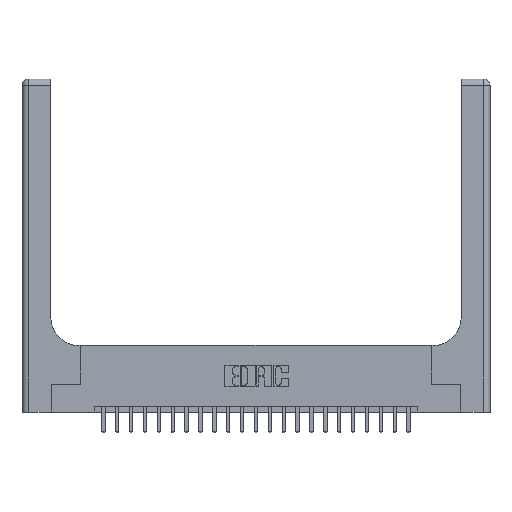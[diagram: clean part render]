
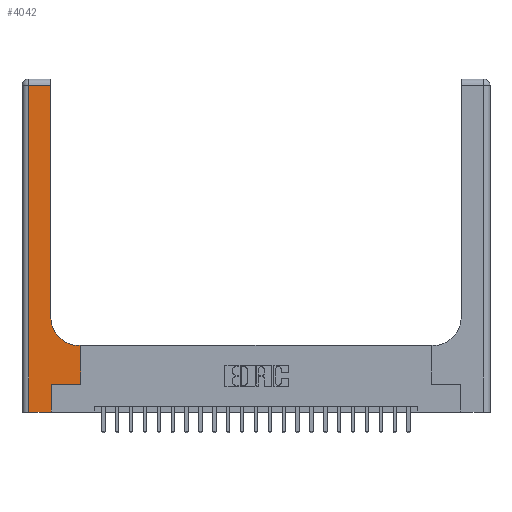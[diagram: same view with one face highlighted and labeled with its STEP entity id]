
A CAD part, top view. The second image highlights one B-rep face of the part: STEP entity #4042.
In plain terms, the highlighted planar face has unit normal (0, 0, 1).
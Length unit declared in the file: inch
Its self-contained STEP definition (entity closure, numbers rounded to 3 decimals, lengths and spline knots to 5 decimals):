
#27 = VECTOR ( 'NONE', #7904, 39.37008 ) ;
#852 = CIRCLE ( 'NONE', #19042, 0.25 ) ;
#1486 = DIRECTION ( 'NONE',  ( 0., 1., 0. ) ) ;
#1932 = VECTOR ( 'NONE', #16519, 39.37008 ) ;
#2194 = VERTEX_POINT ( 'NONE', #18377 ) ;
#3219 = EDGE_CURVE ( 'NONE', #16636, #12512, #12158, .T. ) ;
#3238 = CARTESIAN_POINT ( 'NONE',  ( 0.265, 0.25, 0.37 ) ) ;
#3421 = ORIENTED_EDGE ( 'NONE', *, *, #3219, .T. ) ;
#3640 = EDGE_CURVE ( 'NONE', #7002, #20858, #6030, .T. ) ;
#4042 = ADVANCED_FACE ( 'NONE', ( #11584 ), #17151, .F. ) ;
#4118 = LINE ( 'NONE', #19984, #21814 ) ;
#4289 = VERTEX_POINT ( 'NONE', #11002 ) ;
#4406 = EDGE_CURVE ( 'NONE', #20858, #2194, #7497, .T. ) ;
#4600 = ORIENTED_EDGE ( 'NONE', *, *, #18508, .T. ) ;
#5832 = EDGE_CURVE ( 'NONE', #9207, #16636, #9488, .T. ) ;
#6030 = LINE ( 'NONE', #20322, #13240 ) ;
#6304 = CARTESIAN_POINT ( 'NONE',  ( 0.26, 2.94, 0.37 ) ) ;
#6458 = EDGE_LOOP ( 'NONE', ( #6975, #19548, #4600, #14078, #3421, #20620, #15564, #19941, #20257 ) ) ;
#6661 = CARTESIAN_POINT ( 'NONE',  ( 0.51, 0.6, 0.37 ) ) ;
#6876 = DIRECTION ( 'NONE',  ( 0., 0., -1. ) ) ;
#6975 = ORIENTED_EDGE ( 'NONE', *, *, #3640, .T. ) ;
#7002 = VERTEX_POINT ( 'NONE', #18946 ) ;
#7411 = VECTOR ( 'NONE', #1486, 39.37008 ) ;
#7459 = CARTESIAN_POINT ( 'NONE',  ( 0.528, 0.25, 0.37 ) ) ;
#7497 = LINE ( 'NONE', #13382, #27 ) ;
#7904 = DIRECTION ( 'NONE',  ( -1., 0., 0. ) ) ;
#8096 = EDGE_CURVE ( 'NONE', #19724, #7002, #852, .T. ) ;
#8103 = CARTESIAN_POINT ( 'NONE',  ( 0.265, 0., 0.37 ) ) ;
#8430 = DIRECTION ( 'NONE',  ( 1., 0., 0. ) ) ;
#8785 = EDGE_CURVE ( 'NONE', #4289, #9884, #14945, .T. ) ;
#9207 = VERTEX_POINT ( 'NONE', #20978 ) ;
#9488 = LINE ( 'NONE', #16812, #22719 ) ;
#9552 = EDGE_CURVE ( 'NONE', #9884, #19724, #4118, .T. ) ;
#9756 = DIRECTION ( 'NONE',  ( 1., 0., 0. ) ) ;
#9884 = VERTEX_POINT ( 'NONE', #17939 ) ;
#10251 = CARTESIAN_POINT ( 'NONE',  ( 0.06, 3., 0.37 ) ) ;
#10620 = CARTESIAN_POINT ( 'NONE',  ( 0.265, 0., 0.37 ) ) ;
#11002 = CARTESIAN_POINT ( 'NONE',  ( 0.528, 0.25, 0.37 ) ) ;
#11259 = DIRECTION ( 'NONE',  ( -1., 0., 0. ) ) ;
#11572 = LINE ( 'NONE', #22709, #21508 ) ;
#11584 = FACE_OUTER_BOUND ( 'NONE', #6458, .T. ) ;
#11703 = DIRECTION ( 'NONE',  ( 0., 0., -1. ) ) ;
#12158 = LINE ( 'NONE', #10620, #7411 ) ;
#12384 = LINE ( 'NONE', #10251, #20378 ) ;
#12512 = VERTEX_POINT ( 'NONE', #3238 ) ;
#12918 = AXIS2_PLACEMENT_3D ( 'NONE', #17082, #11703, #20648 ) ;
#13240 = VECTOR ( 'NONE', #18225, 39.37008 ) ;
#13382 = CARTESIAN_POINT ( 'NONE',  ( 0., 2.94, 0.37 ) ) ;
#13654 = DIRECTION ( 'NONE',  ( 0., -1., 0. ) ) ;
#14078 = ORIENTED_EDGE ( 'NONE', *, *, #5832, .T. ) ;
#14945 = LINE ( 'NONE', #7459, #1932 ) ;
#15564 = ORIENTED_EDGE ( 'NONE', *, *, #8785, .T. ) ;
#15713 = CARTESIAN_POINT ( 'NONE',  ( 0.51, 0.85, 0.37 ) ) ;
#16519 = DIRECTION ( 'NONE',  ( 0., 1., 0. ) ) ;
#16636 = VERTEX_POINT ( 'NONE', #8103 ) ;
#16812 = CARTESIAN_POINT ( 'NONE',  ( 0., 0., 0.37 ) ) ;
#17082 = CARTESIAN_POINT ( 'NONE',  ( 0., 3., 0.37 ) ) ;
#17151 = PLANE ( 'NONE',  #12918 ) ;
#17939 = CARTESIAN_POINT ( 'NONE',  ( 0.528, 0.6, 0.37 ) ) ;
#18225 = DIRECTION ( 'NONE',  ( 0., 1., 0. ) ) ;
#18377 = CARTESIAN_POINT ( 'NONE',  ( 0.06, 2.94, 0.37 ) ) ;
#18508 = EDGE_CURVE ( 'NONE', #2194, #9207, #12384, .T. ) ;
#18946 = CARTESIAN_POINT ( 'NONE',  ( 0.26, 0.85, 0.37 ) ) ;
#19042 = AXIS2_PLACEMENT_3D ( 'NONE', #15713, #6876, #19282 ) ;
#19282 = DIRECTION ( 'NONE',  ( 1., 0., 0. ) ) ;
#19548 = ORIENTED_EDGE ( 'NONE', *, *, #4406, .T. ) ;
#19724 = VERTEX_POINT ( 'NONE', #6661 ) ;
#19941 = ORIENTED_EDGE ( 'NONE', *, *, #9552, .T. ) ;
#19984 = CARTESIAN_POINT ( 'NONE',  ( 0.26, 0.6, 0.37 ) ) ;
#20257 = ORIENTED_EDGE ( 'NONE', *, *, #8096, .T. ) ;
#20322 = CARTESIAN_POINT ( 'NONE',  ( 0.26, 3., 0.37 ) ) ;
#20378 = VECTOR ( 'NONE', #13654, 39.37008 ) ;
#20620 = ORIENTED_EDGE ( 'NONE', *, *, #22743, .T. ) ;
#20648 = DIRECTION ( 'NONE',  ( -1., 0., 0. ) ) ;
#20858 = VERTEX_POINT ( 'NONE', #6304 ) ;
#20978 = CARTESIAN_POINT ( 'NONE',  ( 0.06, 0., 0.37 ) ) ;
#21508 = VECTOR ( 'NONE', #8430, 39.37008 ) ;
#21814 = VECTOR ( 'NONE', #11259, 39.37008 ) ;
#22709 = CARTESIAN_POINT ( 'NONE',  ( 0.265, 0.25, 0.37 ) ) ;
#22719 = VECTOR ( 'NONE', #9756, 39.37008 ) ;
#22743 = EDGE_CURVE ( 'NONE', #12512, #4289, #11572, .T. ) ;
